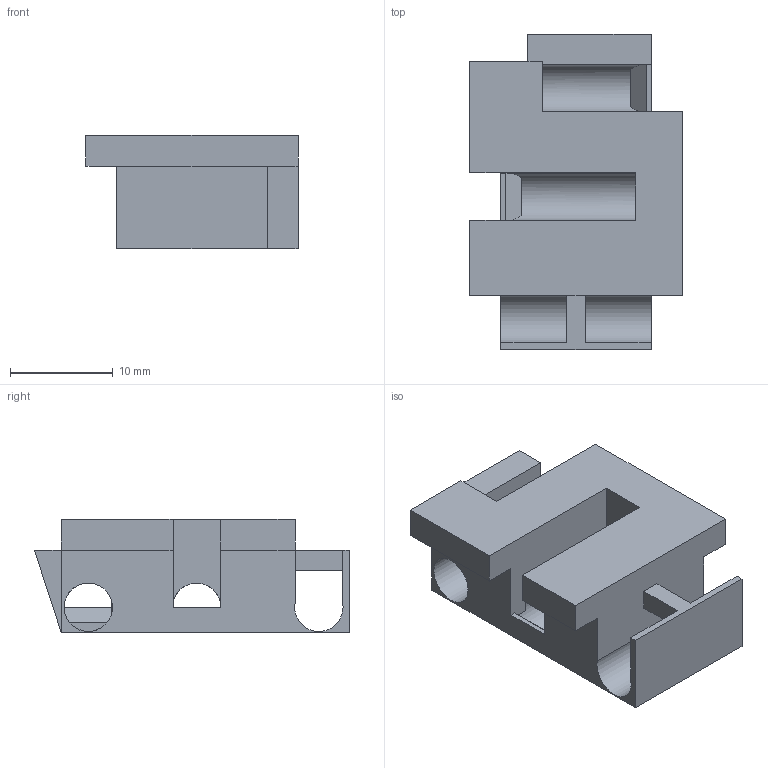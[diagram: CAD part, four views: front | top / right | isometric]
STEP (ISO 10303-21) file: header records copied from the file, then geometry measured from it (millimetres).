
FILE_DESCRIPTION(/* description */ (''),/* implementation_level */ '2;1');
FILE_NAME(/* name */ 'insert_g17_isolated v1.step',/* time_stamp */ '2020-01-05T05:34:02-08:00',/* author */ (''),/* organization */ (''),/* preprocessor_version */ 'ST-DEVELOPER v18',/* originating_system */ 'Autodesk Translation Framework v8.12.0.6',/* authorisation */ '');
FILE_SCHEMA (('AUTOMOTIVE_DESIGN { 1 0 10303 214 3 1 1 }'));
Length unit declared in the file: millimetre
Products named in the file (2): insert_g17_isolated; insert
Assembly tree (1 placements, depth 2):
  insert_g17_isolated
    insert
Bounding box: 20.6 x 30.59 x 11 mm (x, y, z)
Volume: 3059.8 mm3; surface area: 2697.9 mm2
Topology: 1 solids, 1 shells, 45 faces, 135 edges, 89 vertices
Faces by surface type: plane 42, cylinder 3
Full cylindrical faces by diameter (mm): 4.7 x2
Entity records: 1568 total; most frequent: CARTESIAN_POINT 272, ORIENTED_EDGE 270, DIRECTION 249, EDGE_CURVE 135, LINE 117, VECTOR 117, VERTEX_POINT 89, AXIS2_PLACEMENT_3D 66
